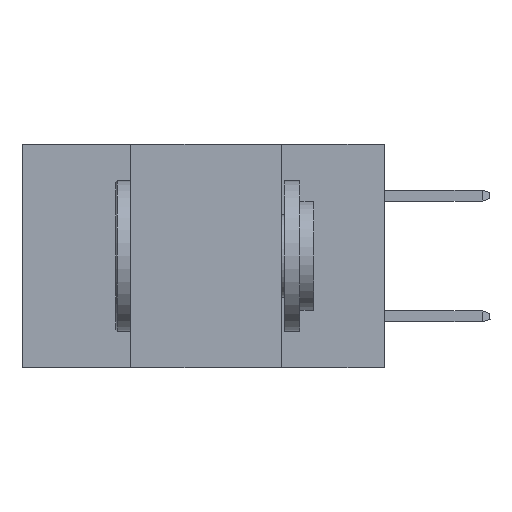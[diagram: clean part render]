
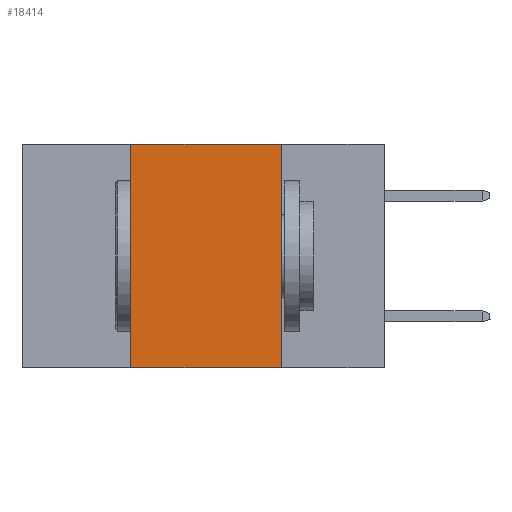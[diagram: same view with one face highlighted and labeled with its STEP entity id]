
A CAD part, left-side view. The second image highlights one B-rep face of the part: STEP entity #18414.
In plain terms, the highlighted planar face has unit normal (-1, 0, 0).
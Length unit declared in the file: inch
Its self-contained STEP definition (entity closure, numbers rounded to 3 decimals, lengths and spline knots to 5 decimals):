
#331 = VECTOR ( 'NONE', #23716, 39.37008 ) ;
#540 = CARTESIAN_POINT ( 'NONE',  ( 0., 0.6, -0.37 ) ) ;
#846 = ORIENTED_EDGE ( 'NONE', *, *, #8319, .F. ) ;
#4242 = VECTOR ( 'NONE', #6212, 39.37008 ) ;
#5176 = DIRECTION ( 'NONE',  ( 1., 0., 0. ) ) ;
#6212 = DIRECTION ( 'NONE',  ( 0., -1., 0. ) ) ;
#6310 = ORIENTED_EDGE ( 'NONE', *, *, #6650, .T. ) ;
#6650 = EDGE_CURVE ( 'NONE', #7012, #14213, #18936, .T. ) ;
#6998 = CARTESIAN_POINT ( 'NONE',  ( 0., 0.42, 0. ) ) ;
#7012 = VERTEX_POINT ( 'NONE', #7293 ) ;
#7293 = CARTESIAN_POINT ( 'NONE',  ( 0., 0.42, -0.37 ) ) ;
#8319 = EDGE_CURVE ( 'NONE', #7012, #11621, #15598, .T. ) ;
#8810 = DIRECTION ( 'NONE',  ( 0., -1., 0. ) ) ;
#10268 = LINE ( 'NONE', #14920, #15376 ) ;
#10900 = VECTOR ( 'NONE', #8810, 39.37008 ) ;
#11621 = VERTEX_POINT ( 'NONE', #6998 ) ;
#12117 = VERTEX_POINT ( 'NONE', #17702 ) ;
#12797 = CARTESIAN_POINT ( 'NONE',  ( 0., 0.6, 0. ) ) ;
#13868 = EDGE_CURVE ( 'NONE', #11621, #12117, #15392, .T. ) ;
#14213 = VERTEX_POINT ( 'NONE', #15504 ) ;
#14920 = CARTESIAN_POINT ( 'NONE',  ( 0., 0.17, -0.37 ) ) ;
#15376 = VECTOR ( 'NONE', #24488, 39.37008 ) ;
#15392 = LINE ( 'NONE', #22238, #10900 ) ;
#15504 = CARTESIAN_POINT ( 'NONE',  ( 0., 0.17, -0.37 ) ) ;
#15598 = LINE ( 'NONE', #17915, #331 ) ;
#16663 = PLANE ( 'NONE',  #20302 ) ;
#17702 = CARTESIAN_POINT ( 'NONE',  ( 0., 0.17, 0. ) ) ;
#17915 = CARTESIAN_POINT ( 'NONE',  ( 0., 0.42, -0.37 ) ) ;
#18414 = ADVANCED_FACE ( 'NONE', ( #20600 ), #16663, .F. ) ;
#18579 = DIRECTION ( 'NONE',  ( 0., 0., -1. ) ) ;
#18936 = LINE ( 'NONE', #540, #4242 ) ;
#19469 = EDGE_LOOP ( 'NONE', ( #20071, #20932, #846, #6310 ) ) ;
#20071 = ORIENTED_EDGE ( 'NONE', *, *, #20442, .F. ) ;
#20302 = AXIS2_PLACEMENT_3D ( 'NONE', #12797, #5176, #18579 ) ;
#20442 = EDGE_CURVE ( 'NONE', #12117, #14213, #10268, .T. ) ;
#20600 = FACE_OUTER_BOUND ( 'NONE', #19469, .T. ) ;
#20932 = ORIENTED_EDGE ( 'NONE', *, *, #13868, .F. ) ;
#22238 = CARTESIAN_POINT ( 'NONE',  ( 0., 0.6, 0. ) ) ;
#23716 = DIRECTION ( 'NONE',  ( 0., 0., 1. ) ) ;
#24488 = DIRECTION ( 'NONE',  ( 0., 0., -1. ) ) ;
